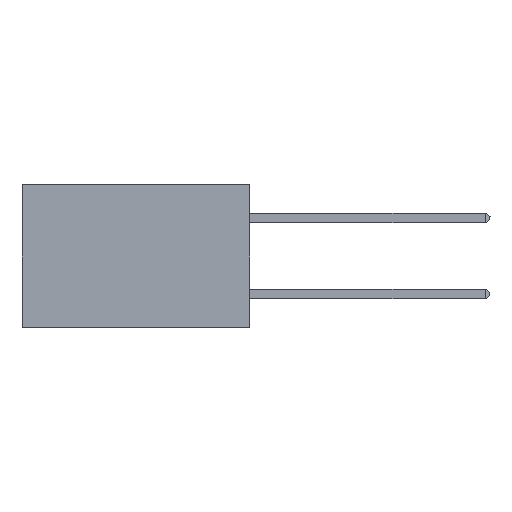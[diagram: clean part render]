
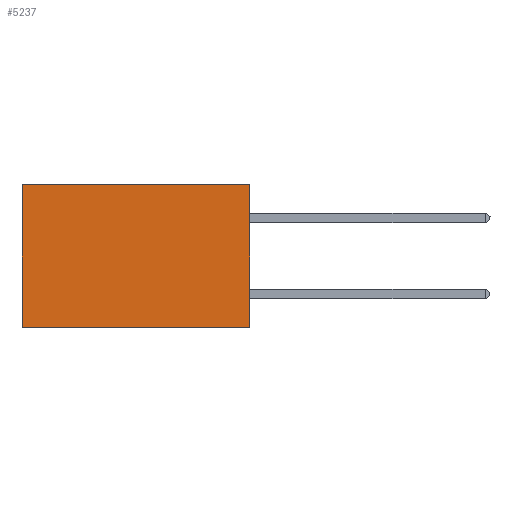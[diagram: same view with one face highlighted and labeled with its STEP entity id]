
A CAD part, left-side view. The second image highlights one B-rep face of the part: STEP entity #5237.
In plain terms, the highlighted planar face has unit normal (-1, 0, 0).
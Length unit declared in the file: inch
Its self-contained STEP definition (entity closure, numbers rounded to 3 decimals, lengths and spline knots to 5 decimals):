
#9 = LINE ( 'NONE', #3702, #6596 ) ;
#840 = EDGE_CURVE ( 'NONE', #1442, #4224, #6441, .T. ) ;
#1033 = DIRECTION ( 'NONE',  ( 0., 0., -1. ) ) ;
#1312 = CARTESIAN_POINT ( 'NONE',  ( 0.2875, 0., -0.375 ) ) ;
#1442 = VERTEX_POINT ( 'NONE', #6387 ) ;
#1683 = ORIENTED_EDGE ( 'NONE', *, *, #4053, .T. ) ;
#1747 = VECTOR ( 'NONE', #5788, 39.37008 ) ;
#1836 = EDGE_CURVE ( 'NONE', #1442, #4777, #9, .T. ) ;
#1910 = CARTESIAN_POINT ( 'NONE',  ( 0.2875, 0., -0.375 ) ) ;
#3120 = VERTEX_POINT ( 'NONE', #6404 ) ;
#3169 = ORIENTED_EDGE ( 'NONE', *, *, #1836, .T. ) ;
#3702 = CARTESIAN_POINT ( 'NONE',  ( 0.2875, 0., 0. ) ) ;
#4053 = EDGE_CURVE ( 'NONE', #4777, #3120, #5991, .T. ) ;
#4172 = VECTOR ( 'NONE', #7617, 39.37008 ) ;
#4187 = AXIS2_PLACEMENT_3D ( 'NONE', #8204, #5699, #7471 ) ;
#4224 = VERTEX_POINT ( 'NONE', #1910 ) ;
#4250 = EDGE_CURVE ( 'NONE', #4224, #3120, #8162, .T. ) ;
#4276 = VECTOR ( 'NONE', #1033, 39.37008 ) ;
#4777 = VERTEX_POINT ( 'NONE', #5272 ) ;
#4956 = PLANE ( 'NONE',  #4187 ) ;
#5038 = DIRECTION ( 'NONE',  ( 0., 1., 0. ) ) ;
#5237 = ADVANCED_FACE ( 'NONE', ( #7030 ), #4956, .F. ) ;
#5272 = CARTESIAN_POINT ( 'NONE',  ( 0.2875, 0.6, 0. ) ) ;
#5423 = ORIENTED_EDGE ( 'NONE', *, *, #840, .F. ) ;
#5699 = DIRECTION ( 'NONE',  ( 1., 0., 0. ) ) ;
#5788 = DIRECTION ( 'NONE',  ( 0., 0., -1. ) ) ;
#5991 = LINE ( 'NONE', #7501, #4276 ) ;
#6387 = CARTESIAN_POINT ( 'NONE',  ( 0.2875, 0., 0. ) ) ;
#6404 = CARTESIAN_POINT ( 'NONE',  ( 0.2875, 0.6, -0.375 ) ) ;
#6441 = LINE ( 'NONE', #1312, #1747 ) ;
#6596 = VECTOR ( 'NONE', #5038, 39.37008 ) ;
#6634 = ORIENTED_EDGE ( 'NONE', *, *, #4250, .F. ) ;
#6994 = CARTESIAN_POINT ( 'NONE',  ( 0.2875, 0., -0.375 ) ) ;
#7030 = FACE_OUTER_BOUND ( 'NONE', #7655, .T. ) ;
#7471 = DIRECTION ( 'NONE',  ( 0., 0., -1. ) ) ;
#7501 = CARTESIAN_POINT ( 'NONE',  ( 0.2875, 0.6, -0.375 ) ) ;
#7617 = DIRECTION ( 'NONE',  ( 0., 1., 0. ) ) ;
#7655 = EDGE_LOOP ( 'NONE', ( #1683, #6634, #5423, #3169 ) ) ;
#8162 = LINE ( 'NONE', #6994, #4172 ) ;
#8204 = CARTESIAN_POINT ( 'NONE',  ( 0.2875, 0., -0.375 ) ) ;
